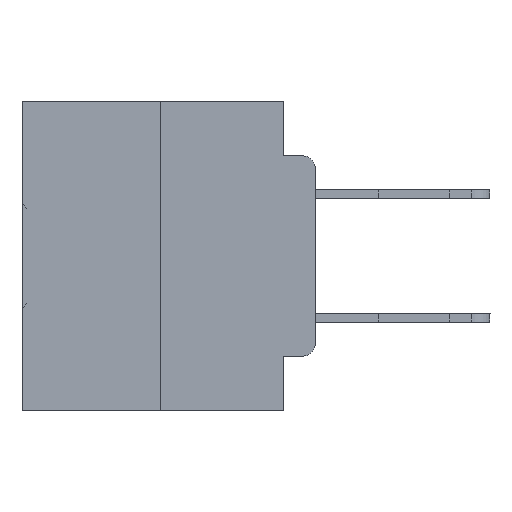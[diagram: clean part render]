
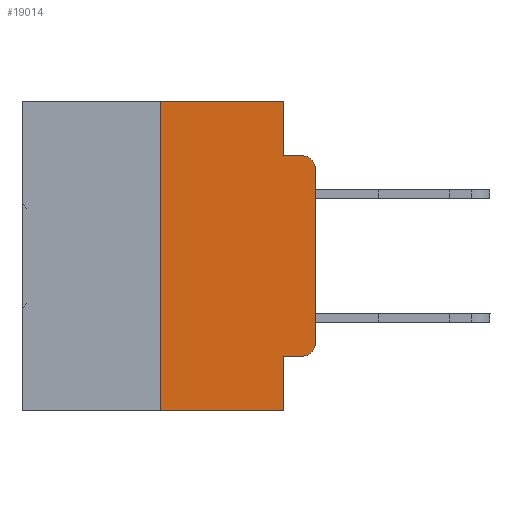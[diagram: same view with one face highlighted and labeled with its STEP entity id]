
A CAD part, left-side view. The second image highlights one B-rep face of the part: STEP entity #19014.
In plain terms, the highlighted planar face has unit normal (-1, 0, 0).
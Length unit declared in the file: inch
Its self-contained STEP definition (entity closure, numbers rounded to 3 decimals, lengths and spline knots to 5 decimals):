
#183 = FACE_OUTER_BOUND ( 'NONE', #7545, .T. ) ;
#1603 = CARTESIAN_POINT ( 'NONE',  ( 0., 0.02, -0.1085 ) ) ;
#2087 = DIRECTION ( 'NONE',  ( 0., 0., -1. ) ) ;
#2102 = EDGE_CURVE ( 'NONE', #7382, #27823, #23663, .T. ) ;
#2479 = CIRCLE ( 'NONE', #2860, 0.02 ) ;
#2521 = VECTOR ( 'NONE', #30667, 39.37008 ) ;
#2860 = AXIS2_PLACEMENT_3D ( 'NONE', #1603, #20545, #28682 ) ;
#3630 = EDGE_CURVE ( 'NONE', #7382, #10385, #33205, .T. ) ;
#3834 = CARTESIAN_POINT ( 'NONE',  ( 0., 0.473, 0. ) ) ;
#4089 = PLANE ( 'NONE',  #17734 ) ;
#4175 = ORIENTED_EDGE ( 'NONE', *, *, #4908, .T. ) ;
#4780 = CARTESIAN_POINT ( 'NONE',  ( 0., 0.051, -0.5 ) ) ;
#4908 = EDGE_CURVE ( 'NONE', #30097, #28829, #2479, .T. ) ;
#5347 = VECTOR ( 'NONE', #30254, 39.37008 ) ;
#5511 = CARTESIAN_POINT ( 'NONE',  ( 0., 0.25, 0. ) ) ;
#5979 = DIRECTION ( 'NONE',  ( 0., -1., 0. ) ) ;
#6807 = DIRECTION ( 'NONE',  ( 0., 0., -1. ) ) ;
#6883 = VERTEX_POINT ( 'NONE', #18149 ) ;
#7186 = EDGE_CURVE ( 'NONE', #33813, #27446, #21251, .T. ) ;
#7234 = VECTOR ( 'NONE', #19129, 39.37008 ) ;
#7331 = ORIENTED_EDGE ( 'NONE', *, *, #2102, .F. ) ;
#7382 = VERTEX_POINT ( 'NONE', #27818 ) ;
#7540 = ORIENTED_EDGE ( 'NONE', *, *, #24252, .F. ) ;
#7545 = EDGE_LOOP ( 'NONE', ( #23586, #4175, #23872, #24084, #7540, #7331, #22096, #12214, #12516, #23038 ) ) ;
#7993 = DIRECTION ( 'NONE',  ( 0., 0., 1. ) ) ;
#8463 = CARTESIAN_POINT ( 'NONE',  ( 0., 0.473, -0.5 ) ) ;
#10385 = VERTEX_POINT ( 'NONE', #4780 ) ;
#11295 = DIRECTION ( 'NONE',  ( 0., -1., 0. ) ) ;
#11500 = EDGE_CURVE ( 'NONE', #11597, #28829, #34904, .T. ) ;
#11597 = VERTEX_POINT ( 'NONE', #34008 ) ;
#11883 = DIRECTION ( 'NONE',  ( 0., 0., 1. ) ) ;
#12022 = CARTESIAN_POINT ( 'NONE',  ( 0., 0.02, -0.0885 ) ) ;
#12214 = ORIENTED_EDGE ( 'NONE', *, *, #31405, .F. ) ;
#12234 = AXIS2_PLACEMENT_3D ( 'NONE', #13137, #15577, #2087 ) ;
#12516 = ORIENTED_EDGE ( 'NONE', *, *, #23717, .T. ) ;
#13137 = CARTESIAN_POINT ( 'NONE',  ( 0., 0.02, -0.3915 ) ) ;
#13911 = LINE ( 'NONE', #14703, #29947 ) ;
#13960 = CARTESIAN_POINT ( 'NONE',  ( 0., 0.051, 0. ) ) ;
#14146 = EDGE_CURVE ( 'NONE', #26280, #11597, #32116, .T. ) ;
#14374 = LINE ( 'NONE', #13960, #7234 ) ;
#14703 = CARTESIAN_POINT ( 'NONE',  ( 0., 0., 0. ) ) ;
#15577 = DIRECTION ( 'NONE',  ( -1., 0., 0. ) ) ;
#15629 = CARTESIAN_POINT ( 'NONE',  ( 0., 0.473, 0. ) ) ;
#15977 = CARTESIAN_POINT ( 'NONE',  ( 0., 0.25, 0. ) ) ;
#16476 = CARTESIAN_POINT ( 'NONE',  ( 0., 0.051, 0. ) ) ;
#17266 = CARTESIAN_POINT ( 'NONE',  ( 0., 0.02, -0.4115 ) ) ;
#17734 = AXIS2_PLACEMENT_3D ( 'NONE', #3834, #33576, #6807 ) ;
#18149 = CARTESIAN_POINT ( 'NONE',  ( 0., 0.051, -0.4115 ) ) ;
#18561 = CARTESIAN_POINT ( 'NONE',  ( 0., 0., -0.3915 ) ) ;
#19014 = ADVANCED_FACE ( 'NONE', ( #183 ), #4089, .F. ) ;
#19129 = DIRECTION ( 'NONE',  ( 0., 0., -1. ) ) ;
#19536 = LINE ( 'NONE', #15629, #25880 ) ;
#20545 = DIRECTION ( 'NONE',  ( -1., 0., 0. ) ) ;
#21251 = CIRCLE ( 'NONE', #12234, 0.02 ) ;
#22096 = ORIENTED_EDGE ( 'NONE', *, *, #3630, .T. ) ;
#22750 = VECTOR ( 'NONE', #5979, 39.37008 ) ;
#23038 = ORIENTED_EDGE ( 'NONE', *, *, #7186, .T. ) ;
#23586 = ORIENTED_EDGE ( 'NONE', *, *, #32777, .T. ) ;
#23663 = LINE ( 'NONE', #5511, #32502 ) ;
#23717 = EDGE_CURVE ( 'NONE', #6883, #33813, #27390, .T. ) ;
#23872 = ORIENTED_EDGE ( 'NONE', *, *, #11500, .F. ) ;
#24084 = ORIENTED_EDGE ( 'NONE', *, *, #14146, .F. ) ;
#24252 = EDGE_CURVE ( 'NONE', #27823, #26280, #19536, .T. ) ;
#25880 = VECTOR ( 'NONE', #34518, 39.37008 ) ;
#26280 = VERTEX_POINT ( 'NONE', #16476 ) ;
#27390 = LINE ( 'NONE', #27569, #22750 ) ;
#27446 = VERTEX_POINT ( 'NONE', #18561 ) ;
#27569 = CARTESIAN_POINT ( 'NONE',  ( 0., 0.051, -0.4115 ) ) ;
#27734 = CARTESIAN_POINT ( 'NONE',  ( 0., 0.051, 0. ) ) ;
#27818 = CARTESIAN_POINT ( 'NONE',  ( 0., 0.25, -0.5 ) ) ;
#27823 = VERTEX_POINT ( 'NONE', #15977 ) ;
#28458 = CARTESIAN_POINT ( 'NONE',  ( 0., 0., -0.1085 ) ) ;
#28682 = DIRECTION ( 'NONE',  ( 0., 0., -1. ) ) ;
#28829 = VERTEX_POINT ( 'NONE', #12022 ) ;
#29947 = VECTOR ( 'NONE', #11883, 39.37008 ) ;
#30097 = VERTEX_POINT ( 'NONE', #28458 ) ;
#30254 = DIRECTION ( 'NONE',  ( 0., -1., 0. ) ) ;
#30667 = DIRECTION ( 'NONE',  ( 0., 0., -1. ) ) ;
#31405 = EDGE_CURVE ( 'NONE', #6883, #10385, #14374, .T. ) ;
#32116 = LINE ( 'NONE', #27734, #2521 ) ;
#32371 = VECTOR ( 'NONE', #11295, 39.37008 ) ;
#32502 = VECTOR ( 'NONE', #7993, 39.37008 ) ;
#32510 = CARTESIAN_POINT ( 'NONE',  ( 0., 0.051, -0.0885 ) ) ;
#32777 = EDGE_CURVE ( 'NONE', #27446, #30097, #13911, .T. ) ;
#33205 = LINE ( 'NONE', #8463, #32371 ) ;
#33576 = DIRECTION ( 'NONE',  ( 1., 0., 0. ) ) ;
#33813 = VERTEX_POINT ( 'NONE', #17266 ) ;
#34008 = CARTESIAN_POINT ( 'NONE',  ( 0., 0.051, -0.0885 ) ) ;
#34518 = DIRECTION ( 'NONE',  ( 0., -1., 0. ) ) ;
#34904 = LINE ( 'NONE', #32510, #5347 ) ;
